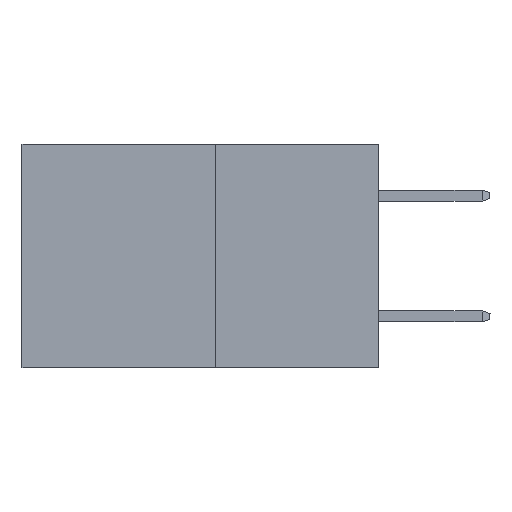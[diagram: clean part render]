
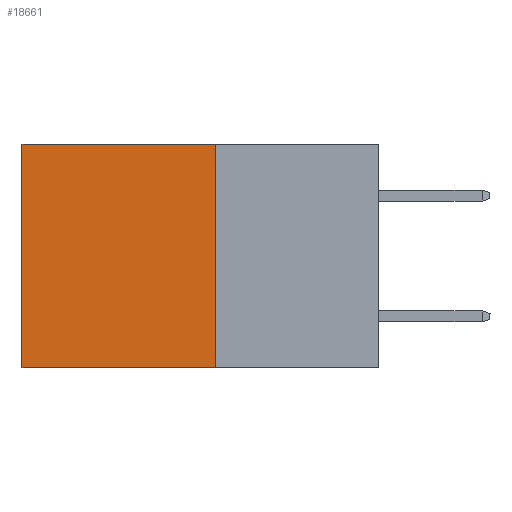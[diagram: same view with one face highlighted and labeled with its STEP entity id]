
A CAD part, left-side view. The second image highlights one B-rep face of the part: STEP entity #18661.
In plain terms, the highlighted planar face has unit normal (-1, 0, 0).
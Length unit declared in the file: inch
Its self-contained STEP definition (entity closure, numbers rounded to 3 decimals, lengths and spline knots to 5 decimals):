
#351 = DIRECTION ( 'NONE',  ( 0., 0., -1. ) ) ;
#1117 = CARTESIAN_POINT ( 'NONE',  ( 0.277, 0.59, -0.37 ) ) ;
#1381 = VERTEX_POINT ( 'NONE', #2009 ) ;
#2009 = CARTESIAN_POINT ( 'NONE',  ( 0.277, 0.27, -0.37 ) ) ;
#2191 = ORIENTED_EDGE ( 'NONE', *, *, #7446, .F. ) ;
#2402 = CARTESIAN_POINT ( 'NONE',  ( 0.277, 0.27, -0.37 ) ) ;
#3488 = VERTEX_POINT ( 'NONE', #13336 ) ;
#4025 = ORIENTED_EDGE ( 'NONE', *, *, #18482, .F. ) ;
#4099 = DIRECTION ( 'NONE',  ( 0., 0., -1. ) ) ;
#4372 = LINE ( 'NONE', #1117, #11918 ) ;
#4978 = CARTESIAN_POINT ( 'NONE',  ( 0.277, 0.27, -0.37 ) ) ;
#6203 = VERTEX_POINT ( 'NONE', #9226 ) ;
#6662 = VECTOR ( 'NONE', #9085, 39.37008 ) ;
#7446 = EDGE_CURVE ( 'NONE', #10201, #1381, #19970, .T. ) ;
#7521 = CARTESIAN_POINT ( 'NONE',  ( 0.277, 0.27, 0. ) ) ;
#8694 = CARTESIAN_POINT ( 'NONE',  ( 0.277, 0.27, -0.37 ) ) ;
#9085 = DIRECTION ( 'NONE',  ( 0., 1., 0. ) ) ;
#9089 = EDGE_LOOP ( 'NONE', ( #20990, #4025, #2191, #11551 ) ) ;
#9226 = CARTESIAN_POINT ( 'NONE',  ( 0.277, 0.59, 0. ) ) ;
#9232 = VECTOR ( 'NONE', #14855, 39.37008 ) ;
#10201 = VERTEX_POINT ( 'NONE', #7521 ) ;
#10326 = DIRECTION ( 'NONE',  ( 1., 0., 0. ) ) ;
#11551 = ORIENTED_EDGE ( 'NONE', *, *, #13864, .T. ) ;
#11918 = VECTOR ( 'NONE', #19307, 39.37008 ) ;
#13083 = LINE ( 'NONE', #4978, #9232 ) ;
#13336 = CARTESIAN_POINT ( 'NONE',  ( 0.277, 0.59, -0.37 ) ) ;
#13864 = EDGE_CURVE ( 'NONE', #10201, #6203, #19235, .T. ) ;
#14598 = VECTOR ( 'NONE', #4099, 39.37008 ) ;
#14855 = DIRECTION ( 'NONE',  ( 0., 1., 0. ) ) ;
#17593 = EDGE_CURVE ( 'NONE', #6203, #3488, #4372, .T. ) ;
#18482 = EDGE_CURVE ( 'NONE', #1381, #3488, #13083, .T. ) ;
#18501 = PLANE ( 'NONE',  #19788 ) ;
#18661 = ADVANCED_FACE ( 'NONE', ( #19227 ), #18501, .F. ) ;
#19227 = FACE_OUTER_BOUND ( 'NONE', #9089, .T. ) ;
#19235 = LINE ( 'NONE', #20525, #6662 ) ;
#19307 = DIRECTION ( 'NONE',  ( 0., 0., -1. ) ) ;
#19788 = AXIS2_PLACEMENT_3D ( 'NONE', #8694, #10326, #351 ) ;
#19970 = LINE ( 'NONE', #2402, #14598 ) ;
#20525 = CARTESIAN_POINT ( 'NONE',  ( 0.277, 0.27, 0. ) ) ;
#20990 = ORIENTED_EDGE ( 'NONE', *, *, #17593, .T. ) ;
